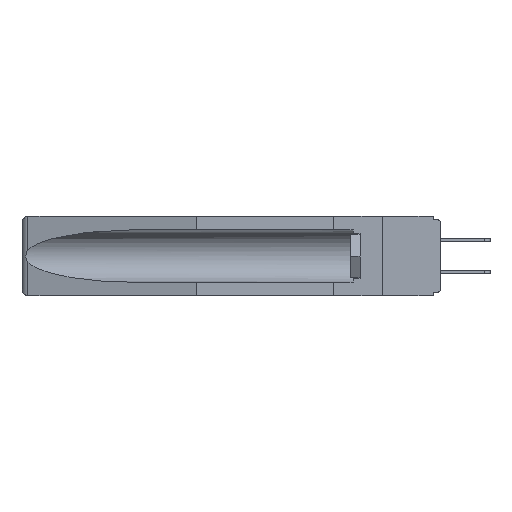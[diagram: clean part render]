
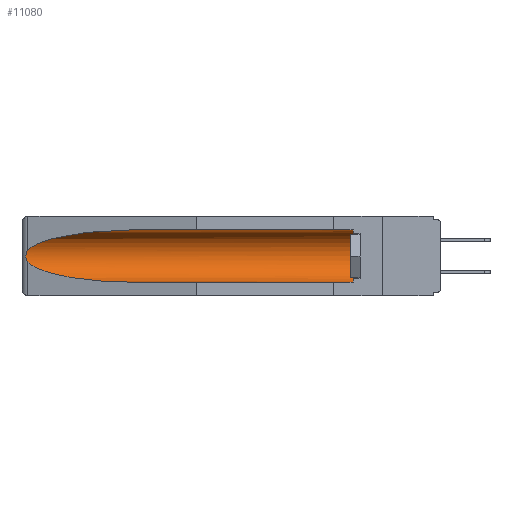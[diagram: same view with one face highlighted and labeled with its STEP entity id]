
A CAD part, left-side view. The second image highlights one B-rep face of the part: STEP entity #11080.
In plain terms, the highlighted cylindrical face has radius 2.857 mm (diameter 5.715 mm), a partial arc.
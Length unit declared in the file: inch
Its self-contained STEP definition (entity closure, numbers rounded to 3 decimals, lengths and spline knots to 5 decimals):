
#449 = ORIENTED_EDGE ( 'NONE', *, *, #1219, .T. ) ;
#860 = CARTESIAN_POINT ( 'NONE',  ( 0.155, 1.07973, -0.284 ) ) ;
#878 = DIRECTION ( 'NONE',  ( 0., 0., 1. ) ) ;
#1219 = EDGE_CURVE ( 'NONE', #17866, #3882, #17170, .T. ) ;
#1795 = CARTESIAN_POINT ( 'NONE',  ( 0.155, -0.30754, -0.059 ) ) ;
#1818 = CARTESIAN_POINT ( 'NONE',  ( 0.2673, 1.5327, -0.16383 ) ) ;
#3882 = VERTEX_POINT ( 'NONE', #19155 ) ;
#4011 = CYLINDRICAL_SURFACE ( 'NONE', #23107, 0.1125 ) ;
#4103 = DIRECTION ( 'NONE',  ( 0., 0., 1. ) ) ;
#4265 = CARTESIAN_POINT ( 'NONE',  ( 0.21114, 1.30732, -0.059 ) ) ;
#4408 = VECTOR ( 'NONE', #10327, 39.37008 ) ;
#4432 = ORIENTED_EDGE ( 'NONE', *, *, #8925, .T. ) ;
#4673 = EDGE_CURVE ( 'NONE', #18366, #17584, #16969, .T. ) ;
#5014 = CARTESIAN_POINT ( 'NONE',  ( 0.25451, 1.48313, -0.09465 ) ) ;
#5094 = CARTESIAN_POINT ( 'NONE',  ( 0.155, 0.126, -0.059 ) ) ;
#5468 = CARTESIAN_POINT ( 'NONE',  ( 0.26654, 1.53092, -0.15636 ) ) ;
#5659 = VERTEX_POINT ( 'NONE', #7499 ) ;
#5664 = ORIENTED_EDGE ( 'NONE', *, *, #23486, .T. ) ;
#5930 = CARTESIAN_POINT ( 'NONE',  ( 0.2675, 1.53308, -0.16763 ) ) ;
#6108 = CARTESIAN_POINT ( 'NONE',  ( 0.26597, 1.5296, -0.19026 ) ) ;
#7076 = EDGE_CURVE ( 'NONE', #7837, #5659, #27145, .T. ) ;
#7499 = CARTESIAN_POINT ( 'NONE',  ( 0.26537, 1.52718, -0.19328 ) ) ;
#7837 = VERTEX_POINT ( 'NONE', #19504 ) ;
#8110 = CARTESIAN_POINT ( 'NONE',  ( 0.155, -0.30754, -0.284 ) ) ;
#8144 = CARTESIAN_POINT ( 'NONE',  ( 0.25451, 1.48313, -0.24835 ) ) ;
#8274 = CARTESIAN_POINT ( 'NONE',  ( 0.2675, 1.53308, -0.17534 ) ) ;
#8925 = EDGE_CURVE ( 'NONE', #5659, #17584, #25466, .T. ) ;
#9028 = EDGE_LOOP ( 'NONE', ( #23031, #20811, #4432, #26393, #5664, #449 ) ) ;
#9419 = CARTESIAN_POINT ( 'NONE',  ( 0.26597, 1.52961, -0.15275 ) ) ;
#9568 = DIRECTION ( 'NONE',  ( 0., -1., 0. ) ) ;
#10072 = CARTESIAN_POINT ( 'NONE',  ( 0.26537, 1.52718, -0.19328 ) ) ;
#10319 = CARTESIAN_POINT ( 'NONE',  ( 0.155, 1.07973, -0.284 ) ) ;
#10327 = DIRECTION ( 'NONE',  ( 0., 1., 0. ) ) ;
#10578 =( BOUNDED_CURVE ( )  B_SPLINE_CURVE ( 3, ( #15718, #4265, #5014, #15534 ),
 .UNSPECIFIED., .F., .F. ) 
 B_SPLINE_CURVE_WITH_KNOTS ( ( 4, 4 ),
 ( 4.71239, 6.08839 ),
 .UNSPECIFIED. ) 
 CURVE ( )  GEOMETRIC_REPRESENTATION_ITEM ( )  RATIONAL_B_SPLINE_CURVE ( ( 1., 0.848, 0.848, 1. ) ) 
 REPRESENTATION_ITEM ( '' )  );
#11080 = ADVANCED_FACE ( 'NONE', ( #20081 ), #4011, .F. ) ;
#14310 = CARTESIAN_POINT ( 'NONE',  ( 0.155, 0.126, -0.284 ) ) ;
#14389 = CIRCLE ( 'NONE', #22613, 0.1125 ) ;
#15534 = CARTESIAN_POINT ( 'NONE',  ( 0.26537, 1.52718, -0.14972 ) ) ;
#15709 = CARTESIAN_POINT ( 'NONE',  ( 0.26537, 1.52718, -0.14972 ) ) ;
#15718 = CARTESIAN_POINT ( 'NONE',  ( 0.155, 1.07973, -0.059 ) ) ;
#15752 = CARTESIAN_POINT ( 'NONE',  ( 0.155, 0.126, -0.1715 ) ) ;
#16272 = EDGE_CURVE ( 'NONE', #3882, #7837, #10578, .T. ) ;
#16707 = CARTESIAN_POINT ( 'NONE',  ( 0.26655, 1.53094, -0.18657 ) ) ;
#16969 = LINE ( 'NONE', #8110, #20961 ) ;
#17170 = LINE ( 'NONE', #1795, #4408 ) ;
#17584 = VERTEX_POINT ( 'NONE', #860 ) ;
#17866 = VERTEX_POINT ( 'NONE', #5094 ) ;
#18366 = VERTEX_POINT ( 'NONE', #14310 ) ;
#19019 = DIRECTION ( 'NONE',  ( 0., 1., 0. ) ) ;
#19155 = CARTESIAN_POINT ( 'NONE',  ( 0.155, 1.07973, -0.059 ) ) ;
#19504 = CARTESIAN_POINT ( 'NONE',  ( 0.26537, 1.52718, -0.14972 ) ) ;
#20081 = FACE_OUTER_BOUND ( 'NONE', #9028, .T. ) ;
#20811 = ORIENTED_EDGE ( 'NONE', *, *, #7076, .T. ) ;
#20884 = CARTESIAN_POINT ( 'NONE',  ( 0.2673, 1.53269, -0.17917 ) ) ;
#20953 = CARTESIAN_POINT ( 'NONE',  ( 0.26537, 1.52718, -0.19328 ) ) ;
#20961 = VECTOR ( 'NONE', #21022, 39.37008 ) ;
#21022 = DIRECTION ( 'NONE',  ( 0., 1., 0. ) ) ;
#22613 = AXIS2_PLACEMENT_3D ( 'NONE', #15752, #9568, #878 ) ;
#23031 = ORIENTED_EDGE ( 'NONE', *, *, #16272, .T. ) ;
#23107 = AXIS2_PLACEMENT_3D ( 'NONE', #27285, #19019, #4103 ) ;
#23486 = EDGE_CURVE ( 'NONE', #18366, #17866, #14389, .T. ) ;
#25064 = CARTESIAN_POINT ( 'NONE',  ( 0.21114, 1.30732, -0.284 ) ) ;
#25466 =( BOUNDED_CURVE ( )  B_SPLINE_CURVE ( 3, ( #20953, #8144, #25064, #10319 ),
 .UNSPECIFIED., .F., .F. ) 
 B_SPLINE_CURVE_WITH_KNOTS ( ( 4, 4 ),
 ( 0.1948, 1.5708 ),
 .UNSPECIFIED. ) 
 CURVE ( )  GEOMETRIC_REPRESENTATION_ITEM ( )  RATIONAL_B_SPLINE_CURVE ( ( 1., 0.848, 0.848, 1. ) ) 
 REPRESENTATION_ITEM ( '' )  );
#26393 = ORIENTED_EDGE ( 'NONE', *, *, #4673, .F. ) ;
#27145 = B_SPLINE_CURVE_WITH_KNOTS ( 'NONE', 3,
 ( #15709, #9419, #5468, #1818, #5930, #8274, #20884, #16707, #6108, #10072 ),
 .UNSPECIFIED., .F., .F.,
 ( 4, 2, 2, 2, 4 ),
 ( 0., 0.00029, 0.00058, 0.00087, 0.00117 ),
 .UNSPECIFIED. ) ;
#27285 = CARTESIAN_POINT ( 'NONE',  ( 0.155, -0.30754, -0.1715 ) ) ;
